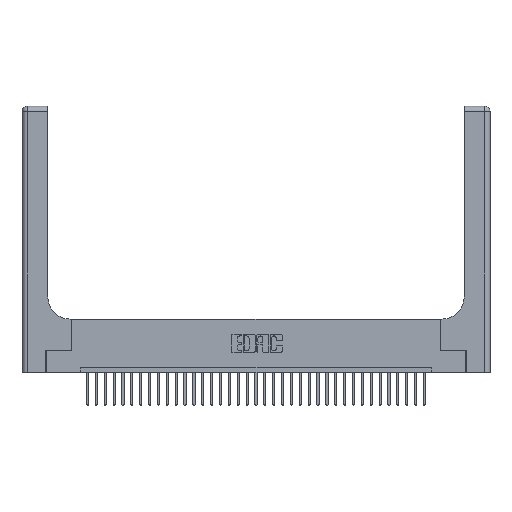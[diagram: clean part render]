
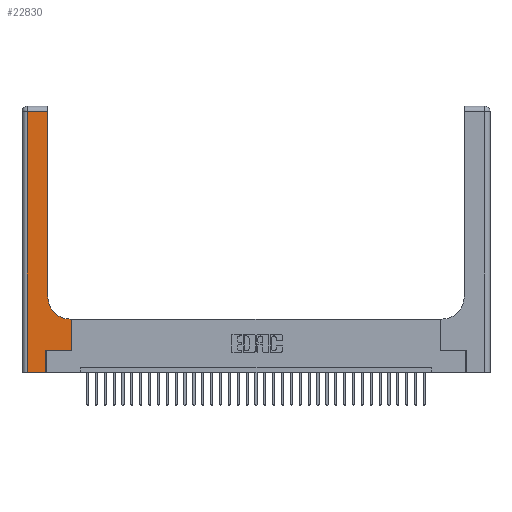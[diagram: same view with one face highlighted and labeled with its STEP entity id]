
A CAD part, top view. The second image highlights one B-rep face of the part: STEP entity #22830.
In plain terms, the highlighted planar face has unit normal (0, 0, 1).
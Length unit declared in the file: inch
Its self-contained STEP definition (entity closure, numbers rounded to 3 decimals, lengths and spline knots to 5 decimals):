
#11 = CARTESIAN_POINT ( 'NONE',  ( 0., 2.94, 0.37 ) ) ;
#272 = EDGE_CURVE ( 'NONE', #10192, #17795, #29199, .T. ) ;
#887 = DIRECTION ( 'NONE',  ( 0., -1., 0. ) ) ;
#1396 = DIRECTION ( 'NONE',  ( 0., 0., -1. ) ) ;
#1648 = FACE_OUTER_BOUND ( 'NONE', #14845, .T. ) ;
#2023 = VERTEX_POINT ( 'NONE', #23504 ) ;
#2345 = VERTEX_POINT ( 'NONE', #14794 ) ;
#2394 = EDGE_CURVE ( 'NONE', #2023, #2345, #5819, .T. ) ;
#3184 = CARTESIAN_POINT ( 'NONE',  ( 0.2915, 3., 0.37 ) ) ;
#3210 = EDGE_CURVE ( 'NONE', #24708, #10192, #34143, .T. ) ;
#3527 = VECTOR ( 'NONE', #887, 39.37008 ) ;
#3600 = CARTESIAN_POINT ( 'NONE',  ( 0.2915, 2.94, 0.37 ) ) ;
#3867 = DIRECTION ( 'NONE',  ( -1., 0., 0. ) ) ;
#5043 = ORIENTED_EDGE ( 'NONE', *, *, #28907, .T. ) ;
#5200 = VECTOR ( 'NONE', #27065, 39.37008 ) ;
#5819 = LINE ( 'NONE', #30524, #18908 ) ;
#6075 = EDGE_CURVE ( 'NONE', #23759, #22475, #6472, .T. ) ;
#6278 = VECTOR ( 'NONE', #32884, 39.37008 ) ;
#6472 = LINE ( 'NONE', #19355, #5200 ) ;
#8136 = CARTESIAN_POINT ( 'NONE',  ( 0.269, 0., 0.37 ) ) ;
#8467 = ORIENTED_EDGE ( 'NONE', *, *, #33791, .T. ) ;
#8931 = DIRECTION ( 'NONE',  ( 0., 0., -1. ) ) ;
#10192 = VERTEX_POINT ( 'NONE', #3600 ) ;
#10800 = VECTOR ( 'NONE', #23257, 39.37008 ) ;
#12416 = ORIENTED_EDGE ( 'NONE', *, *, #30770, .T. ) ;
#12520 = ORIENTED_EDGE ( 'NONE', *, *, #14198, .T. ) ;
#12573 = ORIENTED_EDGE ( 'NONE', *, *, #28709, .T. ) ;
#13179 = CARTESIAN_POINT ( 'NONE',  ( 0.5415, 0.6, 0.37 ) ) ;
#13628 = ORIENTED_EDGE ( 'NONE', *, *, #3210, .T. ) ;
#14198 = EDGE_CURVE ( 'NONE', #27687, #23759, #28033, .T. ) ;
#14344 = CARTESIAN_POINT ( 'NONE',  ( 0.06, 2.94, 0.37 ) ) ;
#14615 = CARTESIAN_POINT ( 'NONE',  ( 0.5585, 0.25, 0.37 ) ) ;
#14794 = CARTESIAN_POINT ( 'NONE',  ( 0.269, 0., 0.37 ) ) ;
#14845 = EDGE_LOOP ( 'NONE', ( #13628, #18632, #5043, #17755, #12573, #12520, #29711, #8467, #12416 ) ) ;
#14957 = CARTESIAN_POINT ( 'NONE',  ( 0.2915, 0.6, 0.37 ) ) ;
#14959 = VERTEX_POINT ( 'NONE', #13179 ) ;
#15080 = DIRECTION ( 'NONE',  ( 1., 0., 0. ) ) ;
#16220 = VECTOR ( 'NONE', #30221, 39.37008 ) ;
#16302 = AXIS2_PLACEMENT_3D ( 'NONE', #17792, #1396, #15080 ) ;
#17289 = CARTESIAN_POINT ( 'NONE',  ( 0.06, 3., 0.37 ) ) ;
#17755 = ORIENTED_EDGE ( 'NONE', *, *, #2394, .T. ) ;
#17792 = CARTESIAN_POINT ( 'NONE',  ( 0.5415, 0.85, 0.37 ) ) ;
#17795 = VERTEX_POINT ( 'NONE', #14344 ) ;
#18632 = ORIENTED_EDGE ( 'NONE', *, *, #272, .T. ) ;
#18883 = CARTESIAN_POINT ( 'NONE',  ( 0.5585, 0.6, 0.37 ) ) ;
#18908 = VECTOR ( 'NONE', #33980, 39.37008 ) ;
#19355 = CARTESIAN_POINT ( 'NONE',  ( 0.5585, 0.25, 0.37 ) ) ;
#20007 = CARTESIAN_POINT ( 'NONE',  ( 0., 3., 0.37 ) ) ;
#20662 = CARTESIAN_POINT ( 'NONE',  ( 0.269, 0.25, 0.37 ) ) ;
#22349 = DIRECTION ( 'NONE',  ( -1., 0., 0. ) ) ;
#22475 = VERTEX_POINT ( 'NONE', #18883 ) ;
#22830 = ADVANCED_FACE ( 'NONE', ( #1648 ), #30602, .F. ) ;
#23163 = CARTESIAN_POINT ( 'NONE',  ( 0.269, 0.25, 0.37 ) ) ;
#23257 = DIRECTION ( 'NONE',  ( 1., 0., 0. ) ) ;
#23504 = CARTESIAN_POINT ( 'NONE',  ( 0.06, 0., 0.37 ) ) ;
#23602 = AXIS2_PLACEMENT_3D ( 'NONE', #20007, #8931, #22349 ) ;
#23759 = VERTEX_POINT ( 'NONE', #14615 ) ;
#24708 = VERTEX_POINT ( 'NONE', #29045 ) ;
#24802 = VECTOR ( 'NONE', #3867, 39.37008 ) ;
#27065 = DIRECTION ( 'NONE',  ( 0., 1., 0. ) ) ;
#27687 = VERTEX_POINT ( 'NONE', #23163 ) ;
#28033 = LINE ( 'NONE', #20662, #10800 ) ;
#28433 = LINE ( 'NONE', #17289, #3527 ) ;
#28709 = EDGE_CURVE ( 'NONE', #2345, #27687, #34376, .T. ) ;
#28907 = EDGE_CURVE ( 'NONE', #17795, #2023, #28433, .T. ) ;
#29045 = CARTESIAN_POINT ( 'NONE',  ( 0.2915, 0.85, 0.37 ) ) ;
#29199 = LINE ( 'NONE', #11, #32964 ) ;
#29711 = ORIENTED_EDGE ( 'NONE', *, *, #6075, .T. ) ;
#30221 = DIRECTION ( 'NONE',  ( 0., 1., 0. ) ) ;
#30524 = CARTESIAN_POINT ( 'NONE',  ( 0., 0., 0.37 ) ) ;
#30602 = PLANE ( 'NONE',  #23602 ) ;
#30770 = EDGE_CURVE ( 'NONE', #14959, #24708, #30916, .T. ) ;
#30916 = CIRCLE ( 'NONE', #16302, 0.25 ) ;
#31627 = LINE ( 'NONE', #14957, #24802 ) ;
#32434 = DIRECTION ( 'NONE',  ( -1., 0., 0. ) ) ;
#32884 = DIRECTION ( 'NONE',  ( 0., 1., 0. ) ) ;
#32964 = VECTOR ( 'NONE', #32434, 39.37008 ) ;
#33791 = EDGE_CURVE ( 'NONE', #22475, #14959, #31627, .T. ) ;
#33980 = DIRECTION ( 'NONE',  ( 1., 0., 0. ) ) ;
#34143 = LINE ( 'NONE', #3184, #6278 ) ;
#34376 = LINE ( 'NONE', #8136, #16220 ) ;
